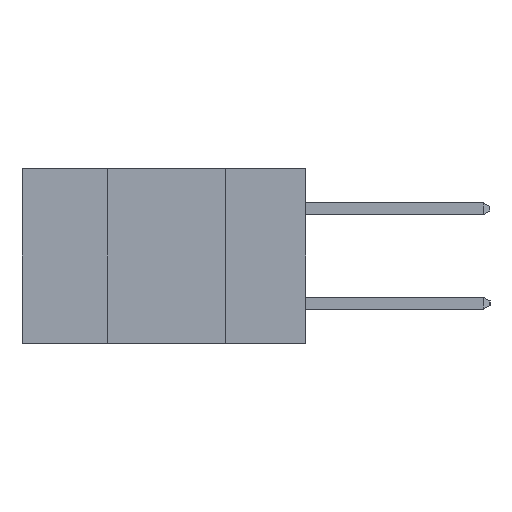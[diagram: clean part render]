
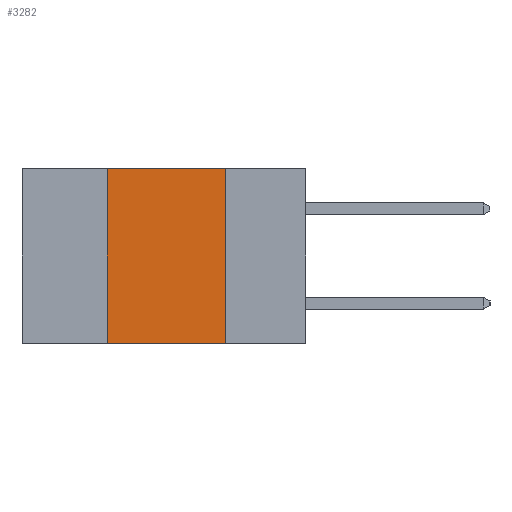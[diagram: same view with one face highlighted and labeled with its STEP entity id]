
A CAD part, left-side view. The second image highlights one B-rep face of the part: STEP entity #3282.
In plain terms, the highlighted planar face has unit normal (-1, 0, 0).
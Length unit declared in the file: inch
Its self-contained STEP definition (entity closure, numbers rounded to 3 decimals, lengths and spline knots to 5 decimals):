
#298 = ORIENTED_EDGE ( 'NONE', *, *, #2396, .F. ) ;
#637 = VECTOR ( 'NONE', #4532, 39.37008 ) ;
#1121 = EDGE_CURVE ( 'NONE', #7202, #2722, #2273, .T. ) ;
#1159 = CARTESIAN_POINT ( 'NONE',  ( 0., 0.17, -0.37 ) ) ;
#1576 = VECTOR ( 'NONE', #7661, 39.37008 ) ;
#2099 = VECTOR ( 'NONE', #10102, 39.37008 ) ;
#2273 = LINE ( 'NONE', #14198, #14308 ) ;
#2396 = EDGE_CURVE ( 'NONE', #7202, #7649, #6863, .T. ) ;
#2489 = LINE ( 'NONE', #10228, #2099 ) ;
#2722 = VERTEX_POINT ( 'NONE', #1159 ) ;
#3282 = ADVANCED_FACE ( 'NONE', ( #7211 ), #3814, .F. ) ;
#3634 = DIRECTION ( 'NONE',  ( 0., 0., -1. ) ) ;
#3711 = CARTESIAN_POINT ( 'NONE',  ( 0., 0.42, -0.37 ) ) ;
#3814 = PLANE ( 'NONE',  #6305 ) ;
#3976 = DIRECTION ( 'NONE',  ( 1., 0., 0. ) ) ;
#4284 = CARTESIAN_POINT ( 'NONE',  ( 0., 0.6, 0. ) ) ;
#4310 = CARTESIAN_POINT ( 'NONE',  ( 0., 0.42, -0.37 ) ) ;
#4532 = DIRECTION ( 'NONE',  ( 0., 0., 1. ) ) ;
#5822 = ORIENTED_EDGE ( 'NONE', *, *, #6621, .F. ) ;
#6305 = AXIS2_PLACEMENT_3D ( 'NONE', #4284, #3976, #3634 ) ;
#6621 = EDGE_CURVE ( 'NONE', #7649, #12077, #2489, .T. ) ;
#6646 = EDGE_LOOP ( 'NONE', ( #14649, #5822, #298, #9683 ) ) ;
#6863 = LINE ( 'NONE', #4310, #637 ) ;
#7202 = VERTEX_POINT ( 'NONE', #3711 ) ;
#7211 = FACE_OUTER_BOUND ( 'NONE', #6646, .T. ) ;
#7649 = VERTEX_POINT ( 'NONE', #10098 ) ;
#7661 = DIRECTION ( 'NONE',  ( 0., 0., -1. ) ) ;
#7748 = CARTESIAN_POINT ( 'NONE',  ( 0., 0.17, -0.37 ) ) ;
#7851 = CARTESIAN_POINT ( 'NONE',  ( 0., 0.17, 0. ) ) ;
#9683 = ORIENTED_EDGE ( 'NONE', *, *, #1121, .T. ) ;
#10098 = CARTESIAN_POINT ( 'NONE',  ( 0., 0.42, 0. ) ) ;
#10102 = DIRECTION ( 'NONE',  ( 0., -1., 0. ) ) ;
#10228 = CARTESIAN_POINT ( 'NONE',  ( 0., 0.6, 0. ) ) ;
#12077 = VERTEX_POINT ( 'NONE', #7851 ) ;
#12095 = EDGE_CURVE ( 'NONE', #12077, #2722, #13980, .T. ) ;
#13980 = LINE ( 'NONE', #7748, #1576 ) ;
#14198 = CARTESIAN_POINT ( 'NONE',  ( 0., 0.6, -0.37 ) ) ;
#14308 = VECTOR ( 'NONE', #14983, 39.37008 ) ;
#14649 = ORIENTED_EDGE ( 'NONE', *, *, #12095, .F. ) ;
#14983 = DIRECTION ( 'NONE',  ( 0., -1., 0. ) ) ;
